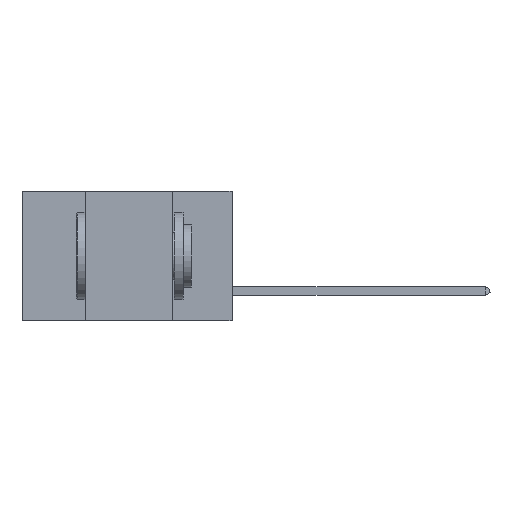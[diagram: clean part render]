
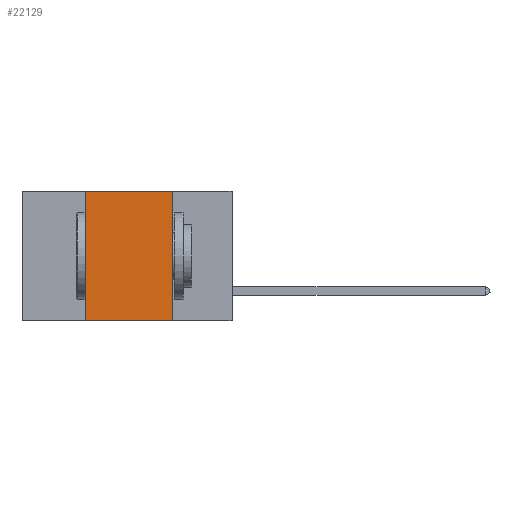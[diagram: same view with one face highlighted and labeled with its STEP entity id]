
A CAD part, left-side view. The second image highlights one B-rep face of the part: STEP entity #22129.
In plain terms, the highlighted planar face has unit normal (-1, 0, 0).
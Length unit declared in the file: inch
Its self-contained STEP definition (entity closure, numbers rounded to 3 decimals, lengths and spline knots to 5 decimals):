
#520 = LINE ( 'NONE', #2759, #14561 ) ;
#891 = CARTESIAN_POINT ( 'NONE',  ( 0., 0.42, 0. ) ) ;
#2660 = LINE ( 'NONE', #17514, #5231 ) ;
#2759 = CARTESIAN_POINT ( 'NONE',  ( 0., 0.42, 0. ) ) ;
#2955 = EDGE_CURVE ( 'NONE', #6608, #7130, #22123, .T. ) ;
#3152 = DIRECTION ( 'NONE',  ( 0., -1., 0. ) ) ;
#4126 = VECTOR ( 'NONE', #5787, 39.37008 ) ;
#5096 = DIRECTION ( 'NONE',  ( 0., 0., -1. ) ) ;
#5231 = VECTOR ( 'NONE', #3152, 39.37008 ) ;
#5553 = CARTESIAN_POINT ( 'NONE',  ( 0., 0.17, 0. ) ) ;
#5787 = DIRECTION ( 'NONE',  ( 0., 0., -1. ) ) ;
#6136 = FACE_OUTER_BOUND ( 'NONE', #9436, .T. ) ;
#6587 = DIRECTION ( 'NONE',  ( 1., 0., 0. ) ) ;
#6608 = VERTEX_POINT ( 'NONE', #891 ) ;
#6840 = EDGE_CURVE ( 'NONE', #7130, #12962, #22935, .T. ) ;
#7130 = VERTEX_POINT ( 'NONE', #13211 ) ;
#7867 = CARTESIAN_POINT ( 'NONE',  ( 0., 0.42, -0.37 ) ) ;
#8432 = CARTESIAN_POINT ( 'NONE',  ( 0., 0.6, 0. ) ) ;
#8771 = ORIENTED_EDGE ( 'NONE', *, *, #17977, .T. ) ;
#9436 = EDGE_LOOP ( 'NONE', ( #19346, #20865, #15369, #8771 ) ) ;
#9810 = VECTOR ( 'NONE', #17428, 39.37008 ) ;
#12962 = VERTEX_POINT ( 'NONE', #12988 ) ;
#12988 = CARTESIAN_POINT ( 'NONE',  ( 0., 0.17, -0.37 ) ) ;
#13211 = CARTESIAN_POINT ( 'NONE',  ( 0., 0.17, 0. ) ) ;
#13470 = DIRECTION ( 'NONE',  ( 0., 0., 1. ) ) ;
#14561 = VECTOR ( 'NONE', #13470, 39.37008 ) ;
#15369 = ORIENTED_EDGE ( 'NONE', *, *, #22506, .F. ) ;
#17428 = DIRECTION ( 'NONE',  ( 0., -1., 0. ) ) ;
#17514 = CARTESIAN_POINT ( 'NONE',  ( 0., 0.6, -0.37 ) ) ;
#17977 = EDGE_CURVE ( 'NONE', #19311, #12962, #2660, .T. ) ;
#19311 = VERTEX_POINT ( 'NONE', #7867 ) ;
#19339 = PLANE ( 'NONE',  #20042 ) ;
#19346 = ORIENTED_EDGE ( 'NONE', *, *, #6840, .F. ) ;
#20042 = AXIS2_PLACEMENT_3D ( 'NONE', #21063, #6587, #5096 ) ;
#20865 = ORIENTED_EDGE ( 'NONE', *, *, #2955, .F. ) ;
#21063 = CARTESIAN_POINT ( 'NONE',  ( 0., 0.6, 0. ) ) ;
#22123 = LINE ( 'NONE', #8432, #9810 ) ;
#22129 = ADVANCED_FACE ( 'NONE', ( #6136 ), #19339, .F. ) ;
#22506 = EDGE_CURVE ( 'NONE', #19311, #6608, #520, .T. ) ;
#22935 = LINE ( 'NONE', #5553, #4126 ) ;
